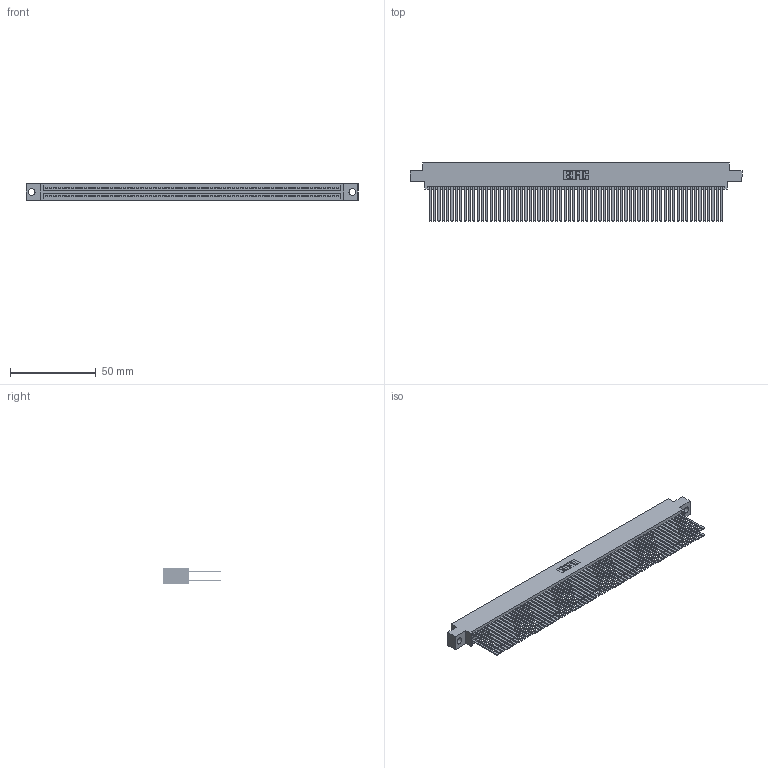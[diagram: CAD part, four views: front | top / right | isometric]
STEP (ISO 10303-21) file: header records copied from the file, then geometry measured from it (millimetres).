
FILE_DESCRIPTION (( 'STEP AP203' ), '1' );
FILE_NAME ('395-136-544-804.STEP', '2021-06-18T02:55:01', ( '' ), ( '' ), 'SwSTEP 2.0', 'SolidWorks 2020', '' );
FILE_SCHEMA (( 'CONFIG_CONTROL_DESIGN' ));
Length unit declared in the file: inch
Products named in the file (3): 395-136-544-804; 345-292-001_345-293-144; 345 Part_0.170 Offset - 0.156 Dia-TI
Assembly tree (137 placements, depth 2):
  395-136-544-804
    345 Part_0.170 Offset - 0.156 Dia-TI
    345-292-001_345-293-144  x136
Bounding box: 193.93 x 33.96 x 9.4 mm (x, y, z)
Volume: 20766.9 mm3; surface area: 36783.3 mm2
Topology: 137 solids, 137 shells, 6128 faces, 18205 edges, 11954 vertices
Faces by surface type: plane 4042, cylinder 2086
Entity records: 50221 total; most frequent: CARTESIAN_POINT 8398, ORIENTED_EDGE 8330, DIRECTION 7369, EDGE_CURVE 4165, VECTOR 3765, LINE 3765, VERTEX_POINT 2774, AXIS2_PLACEMENT_3D 1802
